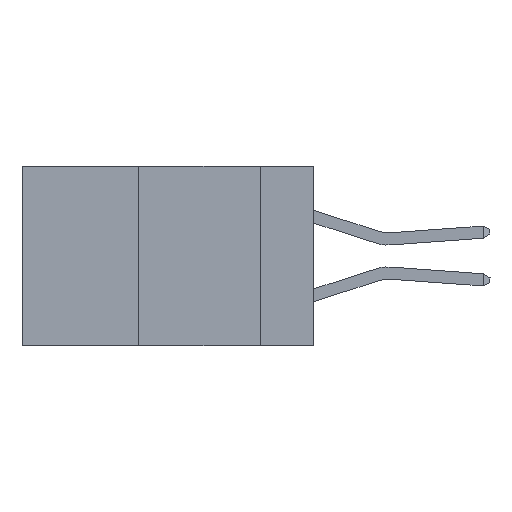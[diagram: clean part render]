
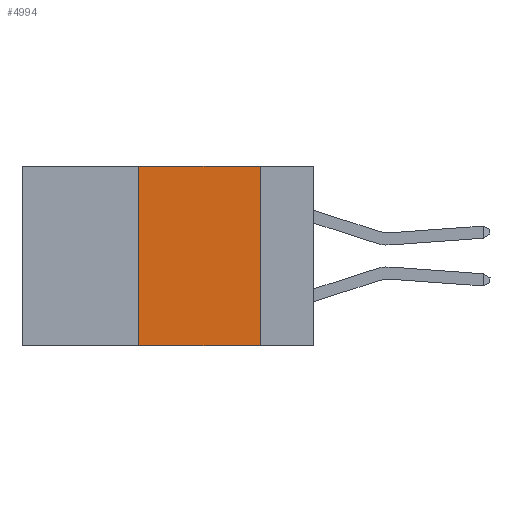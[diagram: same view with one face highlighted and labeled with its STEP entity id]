
A CAD part, left-side view. The second image highlights one B-rep face of the part: STEP entity #4994.
In plain terms, the highlighted planar face has unit normal (-1, 0, 0).
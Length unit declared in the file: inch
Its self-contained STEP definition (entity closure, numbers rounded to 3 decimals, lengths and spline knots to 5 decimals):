
#284 = CARTESIAN_POINT ( 'NONE',  ( 0., 0.36, 0. ) ) ;
#435 = FACE_OUTER_BOUND ( 'NONE', #1932, .T. ) ;
#497 = DIRECTION ( 'NONE',  ( 0., 0., -1. ) ) ;
#624 = CARTESIAN_POINT ( 'NONE',  ( 0., 0.36, 0. ) ) ;
#744 = EDGE_CURVE ( 'NONE', #3403, #14109, #5665, .T. ) ;
#908 = ORIENTED_EDGE ( 'NONE', *, *, #12980, .F. ) ;
#1353 = EDGE_CURVE ( 'NONE', #12220, #11534, #9734, .T. ) ;
#1932 = EDGE_LOOP ( 'NONE', ( #13135, #11175, #908, #12631 ) ) ;
#2557 = CARTESIAN_POINT ( 'NONE',  ( 0., 0.6, -0.37 ) ) ;
#2745 = CARTESIAN_POINT ( 'NONE',  ( 0., 0.36, -0.37 ) ) ;
#3144 = CARTESIAN_POINT ( 'NONE',  ( 0., 0.11, -0.37 ) ) ;
#3246 = VECTOR ( 'NONE', #497, 39.37008 ) ;
#3403 = VERTEX_POINT ( 'NONE', #2745 ) ;
#4451 = LINE ( 'NONE', #624, #17793 ) ;
#4994 = ADVANCED_FACE ( 'NONE', ( #435 ), #13133, .F. ) ;
#5665 = LINE ( 'NONE', #2557, #14789 ) ;
#5873 = CARTESIAN_POINT ( 'NONE',  ( 0., 0.6, 0. ) ) ;
#6193 = DIRECTION ( 'NONE',  ( 0., 0., 1. ) ) ;
#8032 = DIRECTION ( 'NONE',  ( 0., -1., 0. ) ) ;
#8935 = DIRECTION ( 'NONE',  ( 0., -1., 0. ) ) ;
#9707 = CARTESIAN_POINT ( 'NONE',  ( 0., 0.11, 0. ) ) ;
#9734 = LINE ( 'NONE', #5873, #12808 ) ;
#11175 = ORIENTED_EDGE ( 'NONE', *, *, #1353, .F. ) ;
#11534 = VERTEX_POINT ( 'NONE', #9707 ) ;
#12220 = VERTEX_POINT ( 'NONE', #284 ) ;
#12631 = ORIENTED_EDGE ( 'NONE', *, *, #744, .T. ) ;
#12808 = VECTOR ( 'NONE', #8935, 39.37008 ) ;
#12980 = EDGE_CURVE ( 'NONE', #3403, #12220, #4451, .T. ) ;
#13133 = PLANE ( 'NONE',  #16044 ) ;
#13135 = ORIENTED_EDGE ( 'NONE', *, *, #17289, .F. ) ;
#14109 = VERTEX_POINT ( 'NONE', #3144 ) ;
#14789 = VECTOR ( 'NONE', #8032, 39.37008 ) ;
#15648 = CARTESIAN_POINT ( 'NONE',  ( 0., 0.11, 0. ) ) ;
#15955 = DIRECTION ( 'NONE',  ( 1., 0., 0. ) ) ;
#16011 = DIRECTION ( 'NONE',  ( 0., 0., -1. ) ) ;
#16044 = AXIS2_PLACEMENT_3D ( 'NONE', #17371, #15955, #16011 ) ;
#17289 = EDGE_CURVE ( 'NONE', #11534, #14109, #17917, .T. ) ;
#17371 = CARTESIAN_POINT ( 'NONE',  ( 0., 0.6, 0. ) ) ;
#17793 = VECTOR ( 'NONE', #6193, 39.37008 ) ;
#17917 = LINE ( 'NONE', #15648, #3246 ) ;
